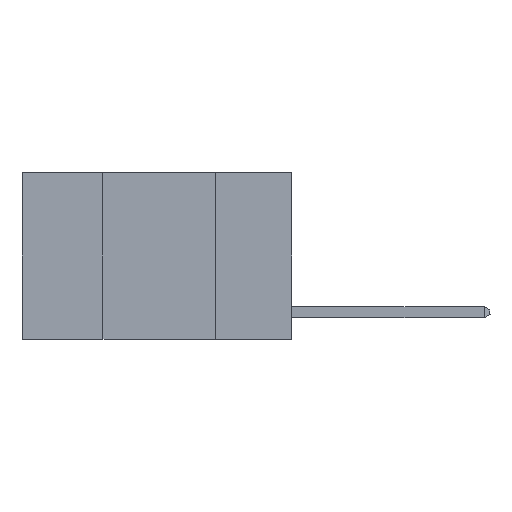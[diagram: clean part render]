
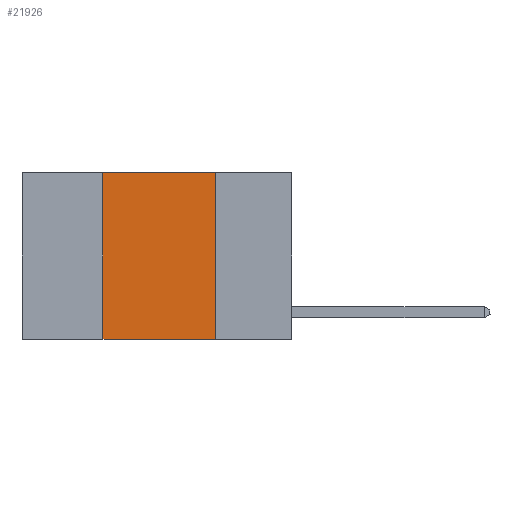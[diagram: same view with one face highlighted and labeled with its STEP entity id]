
A CAD part, left-side view. The second image highlights one B-rep face of the part: STEP entity #21926.
In plain terms, the highlighted planar face has unit normal (-1, 0, 0).
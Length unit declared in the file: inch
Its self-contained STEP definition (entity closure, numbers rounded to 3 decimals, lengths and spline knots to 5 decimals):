
#511 = CARTESIAN_POINT ( 'NONE',  ( 0., 0.6, -0.37 ) ) ;
#763 = VERTEX_POINT ( 'NONE', #2366 ) ;
#1239 = DIRECTION ( 'NONE',  ( 0., 0., -1. ) ) ;
#1890 = LINE ( 'NONE', #17180, #23151 ) ;
#2366 = CARTESIAN_POINT ( 'NONE',  ( 0., 0.42, 0. ) ) ;
#2769 = DIRECTION ( 'NONE',  ( 0., -1., 0. ) ) ;
#3091 = CARTESIAN_POINT ( 'NONE',  ( 0., 0.17, 0. ) ) ;
#3434 = VECTOR ( 'NONE', #13399, 39.37008 ) ;
#4878 = ORIENTED_EDGE ( 'NONE', *, *, #14768, .F. ) ;
#4972 = LINE ( 'NONE', #3091, #7002 ) ;
#5313 = CARTESIAN_POINT ( 'NONE',  ( 0., 0.6, 0. ) ) ;
#6410 = CARTESIAN_POINT ( 'NONE',  ( 0., 0.6, 0. ) ) ;
#7002 = VECTOR ( 'NONE', #1239, 39.37008 ) ;
#7303 = LINE ( 'NONE', #5313, #3434 ) ;
#7406 = EDGE_CURVE ( 'NONE', #14914, #763, #1890, .T. ) ;
#7808 = CARTESIAN_POINT ( 'NONE',  ( 0., 0.42, -0.37 ) ) ;
#8088 = PLANE ( 'NONE',  #22897 ) ;
#9123 = DIRECTION ( 'NONE',  ( 0., 0., 1. ) ) ;
#11278 = EDGE_CURVE ( 'NONE', #17172, #13507, #4972, .T. ) ;
#11378 = ORIENTED_EDGE ( 'NONE', *, *, #11278, .F. ) ;
#12477 = DIRECTION ( 'NONE',  ( 0., 0., -1. ) ) ;
#13399 = DIRECTION ( 'NONE',  ( 0., -1., 0. ) ) ;
#13507 = VERTEX_POINT ( 'NONE', #21706 ) ;
#14070 = DIRECTION ( 'NONE',  ( 1., 0., 0. ) ) ;
#14768 = EDGE_CURVE ( 'NONE', #763, #17172, #7303, .T. ) ;
#14785 = ORIENTED_EDGE ( 'NONE', *, *, #7406, .F. ) ;
#14914 = VERTEX_POINT ( 'NONE', #7808 ) ;
#17172 = VERTEX_POINT ( 'NONE', #20995 ) ;
#17180 = CARTESIAN_POINT ( 'NONE',  ( 0., 0.42, 0. ) ) ;
#18906 = LINE ( 'NONE', #511, #22322 ) ;
#20995 = CARTESIAN_POINT ( 'NONE',  ( 0., 0.17, 0. ) ) ;
#21706 = CARTESIAN_POINT ( 'NONE',  ( 0., 0.17, -0.37 ) ) ;
#21926 = ADVANCED_FACE ( 'NONE', ( #22260 ), #8088, .F. ) ;
#22260 = FACE_OUTER_BOUND ( 'NONE', #24827, .T. ) ;
#22322 = VECTOR ( 'NONE', #2769, 39.37008 ) ;
#22819 = ORIENTED_EDGE ( 'NONE', *, *, #25820, .T. ) ;
#22897 = AXIS2_PLACEMENT_3D ( 'NONE', #6410, #14070, #12477 ) ;
#23151 = VECTOR ( 'NONE', #9123, 39.37008 ) ;
#24827 = EDGE_LOOP ( 'NONE', ( #11378, #4878, #14785, #22819 ) ) ;
#25820 = EDGE_CURVE ( 'NONE', #14914, #13507, #18906, .T. ) ;
